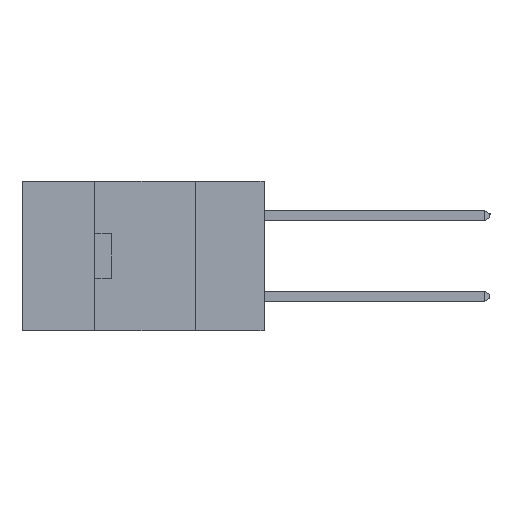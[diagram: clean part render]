
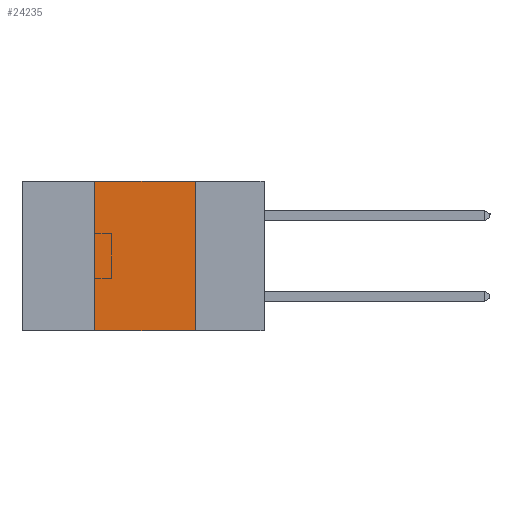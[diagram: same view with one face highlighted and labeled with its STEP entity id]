
A CAD part, left-side view. The second image highlights one B-rep face of the part: STEP entity #24235.
In plain terms, the highlighted planar face has unit normal (-1, 0, 0).
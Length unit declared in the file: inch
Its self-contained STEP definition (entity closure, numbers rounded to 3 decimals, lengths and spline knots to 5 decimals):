
#40 = DIRECTION ( 'NONE',  ( 0., 0., -1. ) ) ;
#223 = EDGE_LOOP ( 'NONE', ( #23225, #16920, #6064, #16810 ) ) ;
#899 = DIRECTION ( 'NONE',  ( 0., -1., 0. ) ) ;
#1335 = VECTOR ( 'NONE', #899, 39.37008 ) ;
#3154 = LINE ( 'NONE', #7257, #1335 ) ;
#3268 = VECTOR ( 'NONE', #19703, 39.37008 ) ;
#3740 = EDGE_CURVE ( 'NONE', #19651, #14219, #10960, .T. ) ;
#5532 = VERTEX_POINT ( 'NONE', #15154 ) ;
#5801 = DIRECTION ( 'NONE',  ( 0., 0., -1. ) ) ;
#6064 = ORIENTED_EDGE ( 'NONE', *, *, #24736, .F. ) ;
#7257 = CARTESIAN_POINT ( 'NONE',  ( 0., 0.6, 0. ) ) ;
#7695 = CARTESIAN_POINT ( 'NONE',  ( 0., 0.42, -0.37 ) ) ;
#8377 = CARTESIAN_POINT ( 'NONE',  ( 0., 0.42, 0. ) ) ;
#9033 = LINE ( 'NONE', #9307, #10785 ) ;
#9307 = CARTESIAN_POINT ( 'NONE',  ( 0., 0.42, -0.37 ) ) ;
#10785 = VECTOR ( 'NONE', #24239, 39.37008 ) ;
#10960 = LINE ( 'NONE', #19832, #3268 ) ;
#11524 = VERTEX_POINT ( 'NONE', #8377 ) ;
#12455 = CARTESIAN_POINT ( 'NONE',  ( 0., 0.17, -0.37 ) ) ;
#12902 = FACE_OUTER_BOUND ( 'NONE', #223, .T. ) ;
#14219 = VERTEX_POINT ( 'NONE', #16661 ) ;
#15095 = VECTOR ( 'NONE', #5801, 39.37008 ) ;
#15154 = CARTESIAN_POINT ( 'NONE',  ( 0., 0.17, 0. ) ) ;
#16661 = CARTESIAN_POINT ( 'NONE',  ( 0., 0.17, -0.37 ) ) ;
#16810 = ORIENTED_EDGE ( 'NONE', *, *, #3740, .T. ) ;
#16920 = ORIENTED_EDGE ( 'NONE', *, *, #23918, .F. ) ;
#17043 = EDGE_CURVE ( 'NONE', #5532, #14219, #25124, .T. ) ;
#19375 = CARTESIAN_POINT ( 'NONE',  ( 0., 0.6, 0. ) ) ;
#19651 = VERTEX_POINT ( 'NONE', #7695 ) ;
#19703 = DIRECTION ( 'NONE',  ( 0., -1., 0. ) ) ;
#19832 = CARTESIAN_POINT ( 'NONE',  ( 0., 0.6, -0.37 ) ) ;
#21499 = PLANE ( 'NONE',  #23436 ) ;
#23225 = ORIENTED_EDGE ( 'NONE', *, *, #17043, .F. ) ;
#23436 = AXIS2_PLACEMENT_3D ( 'NONE', #19375, #25716, #40 ) ;
#23918 = EDGE_CURVE ( 'NONE', #11524, #5532, #3154, .T. ) ;
#24235 = ADVANCED_FACE ( 'NONE', ( #12902 ), #21499, .F. ) ;
#24239 = DIRECTION ( 'NONE',  ( 0., 0., 1. ) ) ;
#24736 = EDGE_CURVE ( 'NONE', #19651, #11524, #9033, .T. ) ;
#25124 = LINE ( 'NONE', #12455, #15095 ) ;
#25716 = DIRECTION ( 'NONE',  ( 1., 0., 0. ) ) ;
